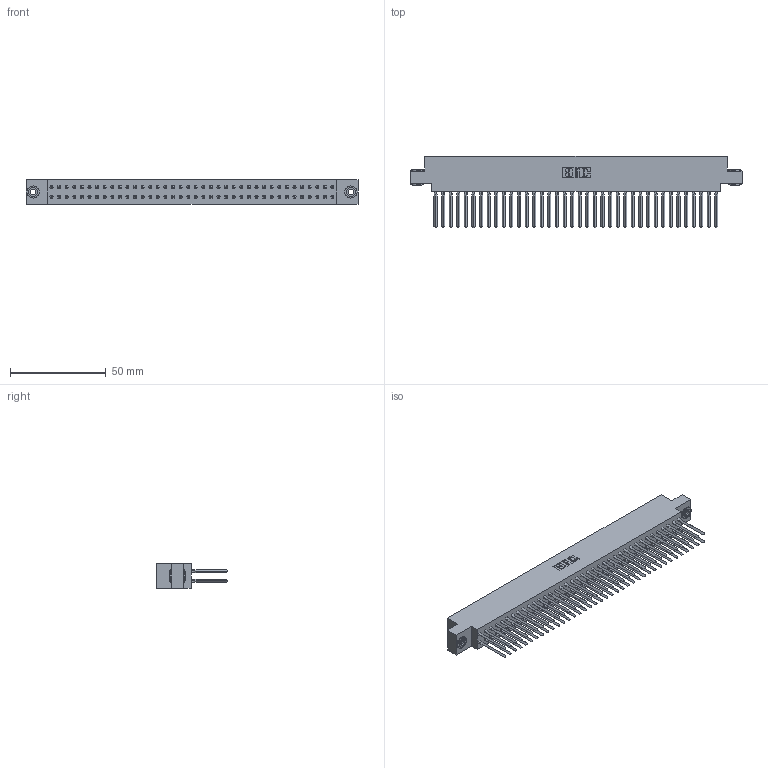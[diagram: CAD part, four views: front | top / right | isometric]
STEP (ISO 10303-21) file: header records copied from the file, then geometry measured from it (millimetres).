
FILE_DESCRIPTION (( 'STEP AP203' ), '1' );
FILE_NAME ('317-076-542-803.STEP', '2020-02-28T08:23:06', ( '' ), ( '' ), 'SwSTEP 2.0', 'SolidWorks 2016', '' );
FILE_SCHEMA (( 'CONFIG_CONTROL_DESIGN' ));
Length unit declared in the file: inch
Products named in the file (4): 345-250-002_345-250-002-102; 317-290-003_542; 317-076-542-803; 317 Part_.156 Dia - TH
Assembly tree (79 placements, depth 2):
  317-076-542-803
    317 Part_.156 Dia - TH
    317-290-003_542  x76
    345-250-002_345-250-002-102  x2
Bounding box: 173.28 x 37.34 x 12.7 mm (x, y, z)
Volume: 28266.8 mm3; surface area: 39395.5 mm2
Topology: 79 solids, 79 shells, 4472 faces, 12511 edges, 7982 vertices
Faces by surface type: plane 3564, cylinder 596, bspline 304, cone 8
Entity records: 55154 total; most frequent: CARTESIAN_POINT 9840, ORIENTED_EDGE 9496, DIRECTION 8034, EDGE_CURVE 4748, VECTOR 4554, LINE 4554, VERTEX_POINT 3158, AXIS2_PLACEMENT_3D 1740
